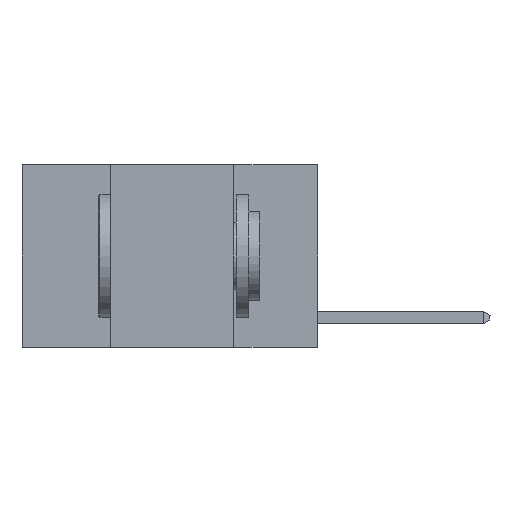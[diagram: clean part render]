
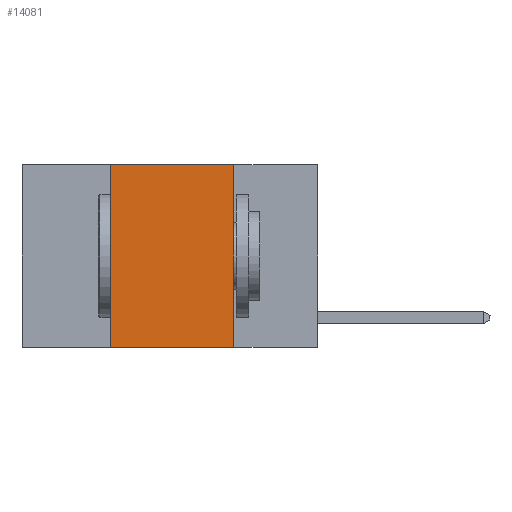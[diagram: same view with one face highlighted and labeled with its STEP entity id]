
A CAD part, left-side view. The second image highlights one B-rep face of the part: STEP entity #14081.
In plain terms, the highlighted planar face has unit normal (-1, 0, 0).
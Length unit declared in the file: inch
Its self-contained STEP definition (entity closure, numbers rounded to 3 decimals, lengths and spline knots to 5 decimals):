
#425 = VERTEX_POINT ( 'NONE', #8893 ) ;
#736 = CARTESIAN_POINT ( 'NONE',  ( 0., 0.6, 0. ) ) ;
#897 = VECTOR ( 'NONE', #11796, 39.37008 ) ;
#1273 = ORIENTED_EDGE ( 'NONE', *, *, #12593, .F. ) ;
#1330 = DIRECTION ( 'NONE',  ( 0., 0., -1. ) ) ;
#1341 = LINE ( 'NONE', #9483, #8796 ) ;
#1927 = ORIENTED_EDGE ( 'NONE', *, *, #16809, .T. ) ;
#2458 = CARTESIAN_POINT ( 'NONE',  ( 0., 0.42, -0.37 ) ) ;
#2513 = CARTESIAN_POINT ( 'NONE',  ( 0., 0.42, 0. ) ) ;
#2708 = LINE ( 'NONE', #16326, #12384 ) ;
#3504 = ORIENTED_EDGE ( 'NONE', *, *, #3776, .F. ) ;
#3776 = EDGE_CURVE ( 'NONE', #9845, #9871, #2708, .T. ) ;
#6901 = PLANE ( 'NONE',  #17332 ) ;
#8302 = CARTESIAN_POINT ( 'NONE',  ( 0., 0.6, 0. ) ) ;
#8399 = EDGE_LOOP ( 'NONE', ( #10027, #1273, #3504, #1927 ) ) ;
#8622 = VERTEX_POINT ( 'NONE', #17542 ) ;
#8796 = VECTOR ( 'NONE', #17386, 39.37008 ) ;
#8893 = CARTESIAN_POINT ( 'NONE',  ( 0., 0.17, 0. ) ) ;
#9483 = CARTESIAN_POINT ( 'NONE',  ( 0., 0.17, 0. ) ) ;
#9512 = LINE ( 'NONE', #12281, #12636 ) ;
#9700 = DIRECTION ( 'NONE',  ( 1., 0., 0. ) ) ;
#9731 = DIRECTION ( 'NONE',  ( 0., 0., 1. ) ) ;
#9845 = VERTEX_POINT ( 'NONE', #2458 ) ;
#9871 = VERTEX_POINT ( 'NONE', #2513 ) ;
#10027 = ORIENTED_EDGE ( 'NONE', *, *, #12094, .F. ) ;
#10683 = FACE_OUTER_BOUND ( 'NONE', #8399, .T. ) ;
#11796 = DIRECTION ( 'NONE',  ( 0., -1., 0. ) ) ;
#11926 = LINE ( 'NONE', #736, #897 ) ;
#12094 = EDGE_CURVE ( 'NONE', #425, #8622, #1341, .T. ) ;
#12281 = CARTESIAN_POINT ( 'NONE',  ( 0., 0.6, -0.37 ) ) ;
#12384 = VECTOR ( 'NONE', #9731, 39.37008 ) ;
#12593 = EDGE_CURVE ( 'NONE', #9871, #425, #11926, .T. ) ;
#12636 = VECTOR ( 'NONE', #14988, 39.37008 ) ;
#14081 = ADVANCED_FACE ( 'NONE', ( #10683 ), #6901, .F. ) ;
#14988 = DIRECTION ( 'NONE',  ( 0., -1., 0. ) ) ;
#16326 = CARTESIAN_POINT ( 'NONE',  ( 0., 0.42, 0. ) ) ;
#16809 = EDGE_CURVE ( 'NONE', #9845, #8622, #9512, .T. ) ;
#17332 = AXIS2_PLACEMENT_3D ( 'NONE', #8302, #9700, #1330 ) ;
#17386 = DIRECTION ( 'NONE',  ( 0., 0., -1. ) ) ;
#17542 = CARTESIAN_POINT ( 'NONE',  ( 0., 0.17, -0.37 ) ) ;
